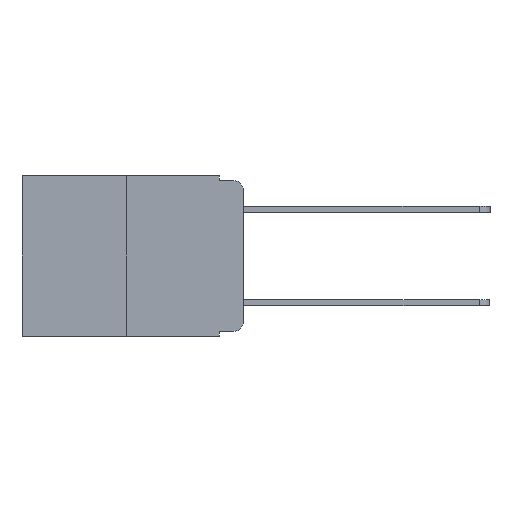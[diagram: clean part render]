
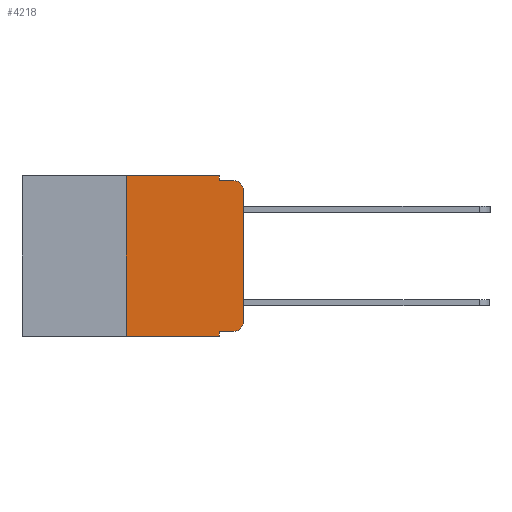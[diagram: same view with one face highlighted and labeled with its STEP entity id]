
A CAD part, left-side view. The second image highlights one B-rep face of the part: STEP entity #4218.
In plain terms, the highlighted planar face has unit normal (-1, 0, 0).
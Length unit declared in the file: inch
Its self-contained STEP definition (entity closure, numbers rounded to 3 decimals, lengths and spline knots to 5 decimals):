
#52 = EDGE_CURVE ( 'NONE', #3005, #4087, #1260, .T. ) ;
#420 = DIRECTION ( 'NONE',  ( 0., -1., 0. ) ) ;
#444 = CARTESIAN_POINT ( 'NONE',  ( 0., 0., 0. ) ) ;
#663 = LINE ( 'NONE', #7054, #9606 ) ;
#1038 = CIRCLE ( 'NONE', #9916, 0.02 ) ;
#1078 = EDGE_LOOP ( 'NONE', ( #4803, #9345, #10740, #8969, #7930, #8653, #8302, #4536, #1624, #6677 ) ) ;
#1260 = LINE ( 'NONE', #8868, #3603 ) ;
#1281 = DIRECTION ( 'NONE',  ( 0., 0., 1. ) ) ;
#1401 = LINE ( 'NONE', #8000, #6203 ) ;
#1445 = VERTEX_POINT ( 'NONE', #5963 ) ;
#1624 = ORIENTED_EDGE ( 'NONE', *, *, #2095, .T. ) ;
#1638 = LINE ( 'NONE', #7363, #6400 ) ;
#2001 = EDGE_CURVE ( 'NONE', #6763, #4087, #663, .T. ) ;
#2095 = EDGE_CURVE ( 'NONE', #6763, #8689, #1401, .T. ) ;
#2592 = AXIS2_PLACEMENT_3D ( 'NONE', #3751, #2844, #5336 ) ;
#2783 = LINE ( 'NONE', #10805, #4977 ) ;
#2844 = DIRECTION ( 'NONE',  ( 1., 0., 0. ) ) ;
#2949 = DIRECTION ( 'NONE',  ( 0., 0., -1. ) ) ;
#3005 = VERTEX_POINT ( 'NONE', #3951 ) ;
#3281 = PLANE ( 'NONE',  #2592 ) ;
#3295 = VECTOR ( 'NONE', #4384, 39.37008 ) ;
#3343 = EDGE_CURVE ( 'NONE', #1445, #7892, #4421, .T. ) ;
#3603 = VECTOR ( 'NONE', #4666, 39.37008 ) ;
#3693 = CARTESIAN_POINT ( 'NONE',  ( 0., 0.051, 0. ) ) ;
#3751 = CARTESIAN_POINT ( 'NONE',  ( 0., 0.473, 0. ) ) ;
#3951 = CARTESIAN_POINT ( 'NONE',  ( 0., 0.25, -0.343 ) ) ;
#3999 = EDGE_CURVE ( 'NONE', #3005, #7212, #2783, .T. ) ;
#4087 = VERTEX_POINT ( 'NONE', #9039 ) ;
#4164 = EDGE_CURVE ( 'NONE', #7892, #9494, #1638, .T. ) ;
#4210 = DIRECTION ( 'NONE',  ( 0., -1., 0. ) ) ;
#4218 = ADVANCED_FACE ( 'NONE', ( #5567 ), #3281, .F. ) ;
#4223 = EDGE_CURVE ( 'NONE', #8689, #6369, #1038, .T. ) ;
#4256 = EDGE_CURVE ( 'NONE', #6369, #8967, #9225, .T. ) ;
#4384 = DIRECTION ( 'NONE',  ( 0., -1., 0. ) ) ;
#4421 = LINE ( 'NONE', #3693, #6561 ) ;
#4447 = CARTESIAN_POINT ( 'NONE',  ( 0., 0.051, -0.01 ) ) ;
#4536 = ORIENTED_EDGE ( 'NONE', *, *, #2001, .F. ) ;
#4666 = DIRECTION ( 'NONE',  ( 0., -1., 0. ) ) ;
#4803 = ORIENTED_EDGE ( 'NONE', *, *, #4256, .T. ) ;
#4894 = DIRECTION ( 'NONE',  ( -1., 0., 0. ) ) ;
#4977 = VECTOR ( 'NONE', #9098, 39.37008 ) ;
#5124 = CARTESIAN_POINT ( 'NONE',  ( 0., 0.02, -0.01 ) ) ;
#5296 = CARTESIAN_POINT ( 'NONE',  ( 0., 0., -0.313 ) ) ;
#5336 = DIRECTION ( 'NONE',  ( 0., 0., -1. ) ) ;
#5567 = FACE_OUTER_BOUND ( 'NONE', #1078, .T. ) ;
#5634 = CARTESIAN_POINT ( 'NONE',  ( 0., 0.25, 0. ) ) ;
#5781 = LINE ( 'NONE', #9905, #3295 ) ;
#5812 = EDGE_CURVE ( 'NONE', #8967, #9494, #6752, .T. ) ;
#5963 = CARTESIAN_POINT ( 'NONE',  ( 0., 0.051, 0. ) ) ;
#5983 = EDGE_CURVE ( 'NONE', #7212, #1445, #5781, .T. ) ;
#6203 = VECTOR ( 'NONE', #4210, 39.37008 ) ;
#6349 = CARTESIAN_POINT ( 'NONE',  ( 0., 0.051, -0.333 ) ) ;
#6369 = VERTEX_POINT ( 'NONE', #5296 ) ;
#6400 = VECTOR ( 'NONE', #420, 39.37008 ) ;
#6561 = VECTOR ( 'NONE', #6787, 39.37008 ) ;
#6677 = ORIENTED_EDGE ( 'NONE', *, *, #4223, .T. ) ;
#6752 = CIRCLE ( 'NONE', #7907, 0.02 ) ;
#6763 = VERTEX_POINT ( 'NONE', #6349 ) ;
#6787 = DIRECTION ( 'NONE',  ( 0., 0., -1. ) ) ;
#7054 = CARTESIAN_POINT ( 'NONE',  ( 0., 0.051, 0. ) ) ;
#7212 = VERTEX_POINT ( 'NONE', #5634 ) ;
#7363 = CARTESIAN_POINT ( 'NONE',  ( 0., 0.051, -0.01 ) ) ;
#7585 = DIRECTION ( 'NONE',  ( -1., 0., 0. ) ) ;
#7607 = CARTESIAN_POINT ( 'NONE',  ( 0., 0.02, -0.313 ) ) ;
#7714 = DIRECTION ( 'NONE',  ( 0., 0., -1. ) ) ;
#7892 = VERTEX_POINT ( 'NONE', #4447 ) ;
#7907 = AXIS2_PLACEMENT_3D ( 'NONE', #9628, #4894, #10288 ) ;
#7930 = ORIENTED_EDGE ( 'NONE', *, *, #5983, .F. ) ;
#8000 = CARTESIAN_POINT ( 'NONE',  ( 0., 0.051, -0.333 ) ) ;
#8302 = ORIENTED_EDGE ( 'NONE', *, *, #52, .T. ) ;
#8653 = ORIENTED_EDGE ( 'NONE', *, *, #3999, .F. ) ;
#8689 = VERTEX_POINT ( 'NONE', #10129 ) ;
#8816 = CARTESIAN_POINT ( 'NONE',  ( 0., 0., -0.03 ) ) ;
#8868 = CARTESIAN_POINT ( 'NONE',  ( 0., 0.473, -0.343 ) ) ;
#8967 = VERTEX_POINT ( 'NONE', #8816 ) ;
#8969 = ORIENTED_EDGE ( 'NONE', *, *, #3343, .F. ) ;
#9039 = CARTESIAN_POINT ( 'NONE',  ( 0., 0.051, -0.343 ) ) ;
#9098 = DIRECTION ( 'NONE',  ( 0., 0., 1. ) ) ;
#9225 = LINE ( 'NONE', #444, #10816 ) ;
#9345 = ORIENTED_EDGE ( 'NONE', *, *, #5812, .T. ) ;
#9494 = VERTEX_POINT ( 'NONE', #5124 ) ;
#9606 = VECTOR ( 'NONE', #2949, 39.37008 ) ;
#9628 = CARTESIAN_POINT ( 'NONE',  ( 0., 0.02, -0.03 ) ) ;
#9905 = CARTESIAN_POINT ( 'NONE',  ( 0., 0.473, 0. ) ) ;
#9916 = AXIS2_PLACEMENT_3D ( 'NONE', #7607, #7585, #7714 ) ;
#10129 = CARTESIAN_POINT ( 'NONE',  ( 0., 0.02, -0.333 ) ) ;
#10288 = DIRECTION ( 'NONE',  ( 0., 0., -1. ) ) ;
#10740 = ORIENTED_EDGE ( 'NONE', *, *, #4164, .F. ) ;
#10805 = CARTESIAN_POINT ( 'NONE',  ( 0., 0.25, 0. ) ) ;
#10816 = VECTOR ( 'NONE', #1281, 39.37008 ) ;
